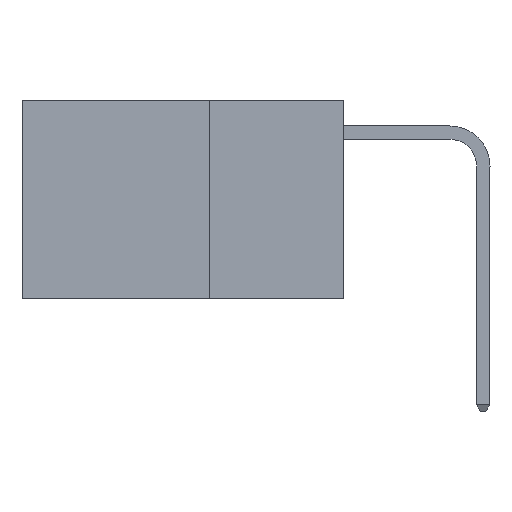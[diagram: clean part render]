
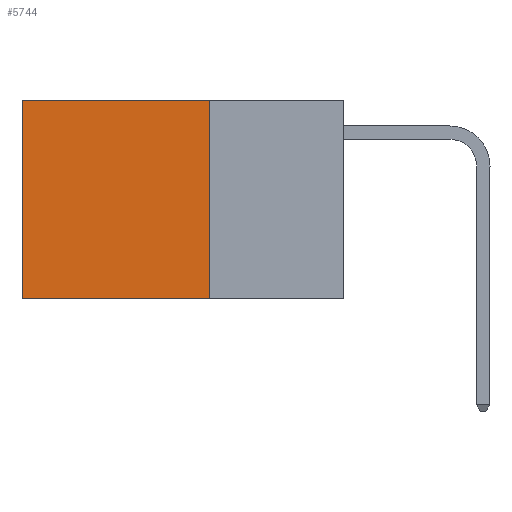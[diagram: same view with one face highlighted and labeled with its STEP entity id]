
A CAD part, left-side view. The second image highlights one B-rep face of the part: STEP entity #5744.
In plain terms, the highlighted planar face has unit normal (-1, 0, 0).
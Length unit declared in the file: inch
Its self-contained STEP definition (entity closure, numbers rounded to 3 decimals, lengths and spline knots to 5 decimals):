
#220 = EDGE_CURVE ( 'NONE', #7306, #3835, #7052, .T. ) ;
#249 = CARTESIAN_POINT ( 'NONE',  ( 0.2625, 0.6, 0. ) ) ;
#298 = DIRECTION ( 'NONE',  ( 0., 0., -1. ) ) ;
#627 = VERTEX_POINT ( 'NONE', #8841 ) ;
#824 = EDGE_CURVE ( 'NONE', #1203, #627, #2290, .T. ) ;
#921 = AXIS2_PLACEMENT_3D ( 'NONE', #3236, #3092, #3079 ) ;
#1101 = LINE ( 'NONE', #8407, #1145 ) ;
#1119 = VECTOR ( 'NONE', #298, 39.37008 ) ;
#1145 = VECTOR ( 'NONE', #8227, 39.37008 ) ;
#1203 = VERTEX_POINT ( 'NONE', #8420 ) ;
#1262 = FACE_OUTER_BOUND ( 'NONE', #6772, .T. ) ;
#1753 = CARTESIAN_POINT ( 'NONE',  ( 0.2625, 0.25, -0.37 ) ) ;
#1776 = VECTOR ( 'NONE', #4918, 39.37008 ) ;
#1830 = CARTESIAN_POINT ( 'NONE',  ( 0.2625, 0.25, 0. ) ) ;
#2290 = LINE ( 'NONE', #1753, #1776 ) ;
#2441 = EDGE_CURVE ( 'NONE', #3835, #627, #6771, .T. ) ;
#2464 = DIRECTION ( 'NONE',  ( 0., 1., 0. ) ) ;
#2540 = CARTESIAN_POINT ( 'NONE',  ( 0.2625, 0.6, 0. ) ) ;
#3079 = DIRECTION ( 'NONE',  ( 0., 0., -1. ) ) ;
#3092 = DIRECTION ( 'NONE',  ( 1., 0., 0. ) ) ;
#3148 = PLANE ( 'NONE',  #921 ) ;
#3236 = CARTESIAN_POINT ( 'NONE',  ( 0.2625, 0.25, 0. ) ) ;
#3647 = EDGE_CURVE ( 'NONE', #7306, #1203, #1101, .T. ) ;
#3835 = VERTEX_POINT ( 'NONE', #2540 ) ;
#4918 = DIRECTION ( 'NONE',  ( 0., 1., 0. ) ) ;
#5744 = ADVANCED_FACE ( 'NONE', ( #1262 ), #3148, .F. ) ;
#6771 = LINE ( 'NONE', #249, #1119 ) ;
#6772 = EDGE_LOOP ( 'NONE', ( #8496, #8715, #7377, #6810 ) ) ;
#6810 = ORIENTED_EDGE ( 'NONE', *, *, #220, .T. ) ;
#6974 = VECTOR ( 'NONE', #2464, 39.37008 ) ;
#7052 = LINE ( 'NONE', #1830, #6974 ) ;
#7306 = VERTEX_POINT ( 'NONE', #8257 ) ;
#7377 = ORIENTED_EDGE ( 'NONE', *, *, #3647, .F. ) ;
#8227 = DIRECTION ( 'NONE',  ( 0., 0., -1. ) ) ;
#8257 = CARTESIAN_POINT ( 'NONE',  ( 0.2625, 0.25, 0. ) ) ;
#8407 = CARTESIAN_POINT ( 'NONE',  ( 0.2625, 0.25, 0. ) ) ;
#8420 = CARTESIAN_POINT ( 'NONE',  ( 0.2625, 0.25, -0.37 ) ) ;
#8496 = ORIENTED_EDGE ( 'NONE', *, *, #2441, .T. ) ;
#8715 = ORIENTED_EDGE ( 'NONE', *, *, #824, .F. ) ;
#8841 = CARTESIAN_POINT ( 'NONE',  ( 0.2625, 0.6, -0.37 ) ) ;
